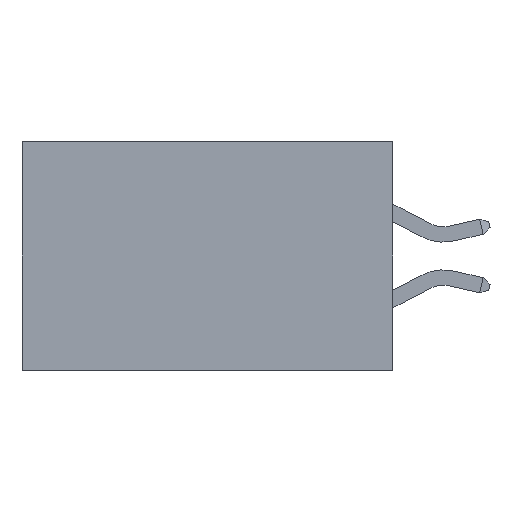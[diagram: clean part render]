
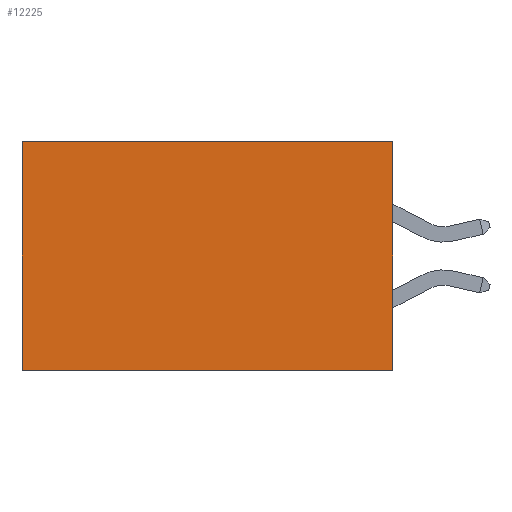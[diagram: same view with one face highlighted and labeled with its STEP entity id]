
A CAD part, left-side view. The second image highlights one B-rep face of the part: STEP entity #12225.
In plain terms, the highlighted planar face has unit normal (-1, 0, 0).
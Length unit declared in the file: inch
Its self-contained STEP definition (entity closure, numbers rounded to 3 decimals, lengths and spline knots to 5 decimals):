
#9 = CARTESIAN_POINT ( 'NONE',  ( 0.2875, 0., -0.37 ) ) ;
#72 = VERTEX_POINT ( 'NONE', #6730 ) ;
#135 = VERTEX_POINT ( 'NONE', #3713 ) ;
#774 = ORIENTED_EDGE ( 'NONE', *, *, #8210, .F. ) ;
#1348 = LINE ( 'NONE', #14152, #13714 ) ;
#1499 = ORIENTED_EDGE ( 'NONE', *, *, #1543, .T. ) ;
#1543 = EDGE_CURVE ( 'NONE', #6895, #135, #5816, .T. ) ;
#1705 = VERTEX_POINT ( 'NONE', #9 ) ;
#2838 = LINE ( 'NONE', #3540, #5332 ) ;
#3006 = DIRECTION ( 'NONE',  ( 1., 0., 0. ) ) ;
#3453 = DIRECTION ( 'NONE',  ( 0., 1., 0. ) ) ;
#3540 = CARTESIAN_POINT ( 'NONE',  ( 0.2875, 0., 0. ) ) ;
#3713 = CARTESIAN_POINT ( 'NONE',  ( 0.2875, 0.6, -0.37 ) ) ;
#4238 = CARTESIAN_POINT ( 'NONE',  ( 0.2875, 0., 0. ) ) ;
#4726 = EDGE_LOOP ( 'NONE', ( #1499, #774, #6294, #7999 ) ) ;
#5105 = VECTOR ( 'NONE', #6658, 39.37008 ) ;
#5332 = VECTOR ( 'NONE', #13097, 39.37008 ) ;
#5430 = PLANE ( 'NONE',  #11671 ) ;
#5816 = LINE ( 'NONE', #9939, #8608 ) ;
#6009 = FACE_OUTER_BOUND ( 'NONE', #4726, .T. ) ;
#6294 = ORIENTED_EDGE ( 'NONE', *, *, #9009, .F. ) ;
#6658 = DIRECTION ( 'NONE',  ( 0., 1., 0. ) ) ;
#6730 = CARTESIAN_POINT ( 'NONE',  ( 0.2875, 0., 0. ) ) ;
#6895 = VERTEX_POINT ( 'NONE', #7029 ) ;
#7029 = CARTESIAN_POINT ( 'NONE',  ( 0.2875, 0.6, 0. ) ) ;
#7999 = ORIENTED_EDGE ( 'NONE', *, *, #10069, .T. ) ;
#8210 = EDGE_CURVE ( 'NONE', #1705, #135, #1348, .T. ) ;
#8608 = VECTOR ( 'NONE', #13983, 39.37008 ) ;
#9009 = EDGE_CURVE ( 'NONE', #72, #1705, #2838, .T. ) ;
#9939 = CARTESIAN_POINT ( 'NONE',  ( 0.2875, 0.6, 0. ) ) ;
#10069 = EDGE_CURVE ( 'NONE', #72, #6895, #14540, .T. ) ;
#11403 = DIRECTION ( 'NONE',  ( 0., 0., -1. ) ) ;
#11671 = AXIS2_PLACEMENT_3D ( 'NONE', #14826, #3006, #11403 ) ;
#12225 = ADVANCED_FACE ( 'NONE', ( #6009 ), #5430, .F. ) ;
#13097 = DIRECTION ( 'NONE',  ( 0., 0., -1. ) ) ;
#13714 = VECTOR ( 'NONE', #3453, 39.37008 ) ;
#13983 = DIRECTION ( 'NONE',  ( 0., 0., -1. ) ) ;
#14152 = CARTESIAN_POINT ( 'NONE',  ( 0.2875, 0., -0.37 ) ) ;
#14540 = LINE ( 'NONE', #4238, #5105 ) ;
#14826 = CARTESIAN_POINT ( 'NONE',  ( 0.2875, 0., 0. ) ) ;
